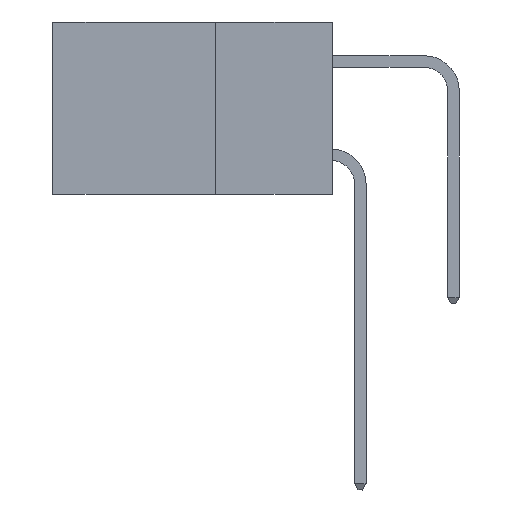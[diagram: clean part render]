
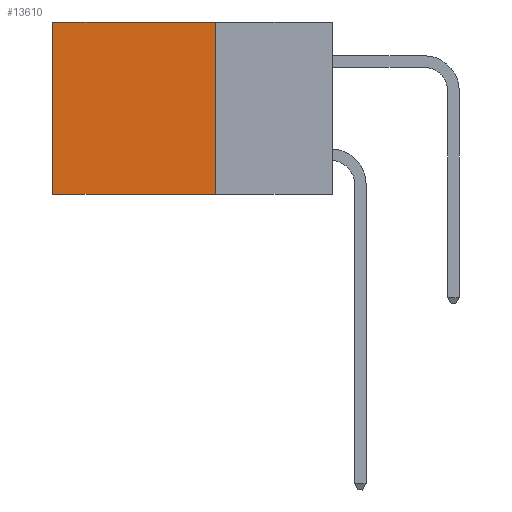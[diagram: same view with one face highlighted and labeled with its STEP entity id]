
A CAD part, left-side view. The second image highlights one B-rep face of the part: STEP entity #13610.
In plain terms, the highlighted planar face has unit normal (-1, 0, 0).
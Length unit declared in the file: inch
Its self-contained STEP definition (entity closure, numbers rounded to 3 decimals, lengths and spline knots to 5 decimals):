
#59 = DIRECTION ( 'NONE',  ( 0., 1., 0. ) ) ;
#495 = EDGE_CURVE ( 'NONE', #11937, #13209, #2542, .T. ) ;
#637 = CARTESIAN_POINT ( 'NONE',  ( 0.298, 0.25, 0. ) ) ;
#958 = EDGE_CURVE ( 'NONE', #15475, #8171, #8647, .T. ) ;
#1938 = CARTESIAN_POINT ( 'NONE',  ( 0.298, 0.25, -0.37 ) ) ;
#2128 = CARTESIAN_POINT ( 'NONE',  ( 0.298, 0.6, 0. ) ) ;
#2542 = LINE ( 'NONE', #2128, #5441 ) ;
#2691 = ORIENTED_EDGE ( 'NONE', *, *, #6666, .F. ) ;
#2808 = DIRECTION ( 'NONE',  ( 0., 0., -1. ) ) ;
#2834 = VECTOR ( 'NONE', #7462, 39.37008 ) ;
#2882 = CARTESIAN_POINT ( 'NONE',  ( 0.298, 0.6, 0. ) ) ;
#3366 = PLANE ( 'NONE',  #14099 ) ;
#4335 = EDGE_CURVE ( 'NONE', #15475, #11937, #6131, .T. ) ;
#4437 = CARTESIAN_POINT ( 'NONE',  ( 0.298, 0.25, 0. ) ) ;
#4591 = DIRECTION ( 'NONE',  ( 1., 0., 0. ) ) ;
#4869 = CARTESIAN_POINT ( 'NONE',  ( 0.298, 0.6, -0.37 ) ) ;
#5414 = DIRECTION ( 'NONE',  ( 0., 0., -1. ) ) ;
#5433 = ORIENTED_EDGE ( 'NONE', *, *, #495, .T. ) ;
#5441 = VECTOR ( 'NONE', #2808, 39.37008 ) ;
#6131 = LINE ( 'NONE', #11683, #2834 ) ;
#6666 = EDGE_CURVE ( 'NONE', #8171, #13209, #8500, .T. ) ;
#7462 = DIRECTION ( 'NONE',  ( 0., 1., 0. ) ) ;
#7593 = FACE_OUTER_BOUND ( 'NONE', #15221, .T. ) ;
#8171 = VERTEX_POINT ( 'NONE', #13343 ) ;
#8488 = ORIENTED_EDGE ( 'NONE', *, *, #4335, .T. ) ;
#8500 = LINE ( 'NONE', #1938, #14457 ) ;
#8647 = LINE ( 'NONE', #4437, #11038 ) ;
#10452 = ORIENTED_EDGE ( 'NONE', *, *, #958, .F. ) ;
#11038 = VECTOR ( 'NONE', #5414, 39.37008 ) ;
#11683 = CARTESIAN_POINT ( 'NONE',  ( 0.298, 0.25, 0. ) ) ;
#11801 = CARTESIAN_POINT ( 'NONE',  ( 0.298, 0.25, 0. ) ) ;
#11937 = VERTEX_POINT ( 'NONE', #2882 ) ;
#13003 = DIRECTION ( 'NONE',  ( 0., 0., -1. ) ) ;
#13209 = VERTEX_POINT ( 'NONE', #4869 ) ;
#13343 = CARTESIAN_POINT ( 'NONE',  ( 0.298, 0.25, -0.37 ) ) ;
#13610 = ADVANCED_FACE ( 'NONE', ( #7593 ), #3366, .F. ) ;
#14099 = AXIS2_PLACEMENT_3D ( 'NONE', #11801, #4591, #13003 ) ;
#14457 = VECTOR ( 'NONE', #59, 39.37008 ) ;
#15221 = EDGE_LOOP ( 'NONE', ( #5433, #2691, #10452, #8488 ) ) ;
#15475 = VERTEX_POINT ( 'NONE', #637 ) ;
